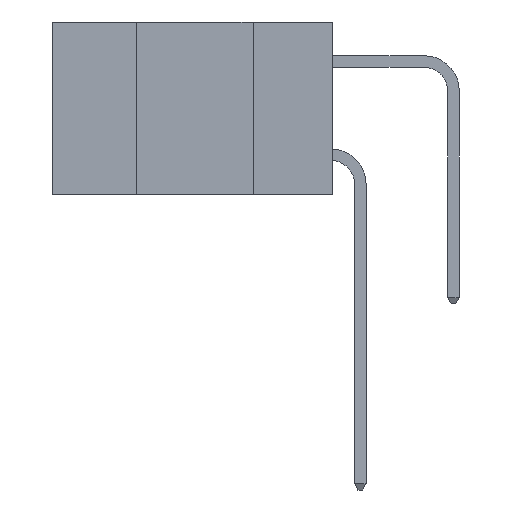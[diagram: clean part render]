
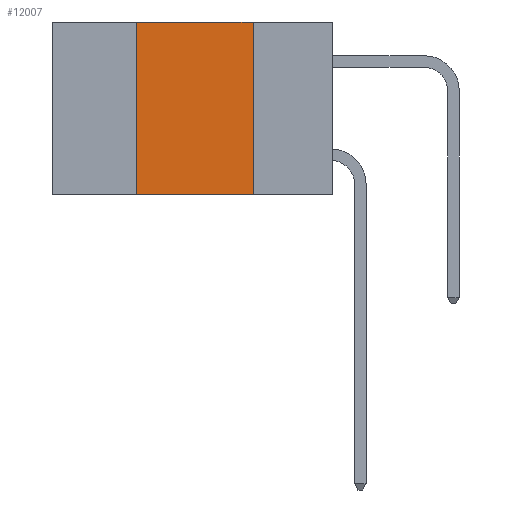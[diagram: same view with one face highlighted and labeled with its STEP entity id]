
A CAD part, left-side view. The second image highlights one B-rep face of the part: STEP entity #12007.
In plain terms, the highlighted planar face has unit normal (-1, 0, 0).
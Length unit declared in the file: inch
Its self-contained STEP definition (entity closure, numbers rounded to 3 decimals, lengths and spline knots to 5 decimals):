
#163 = CARTESIAN_POINT ( 'NONE',  ( 0., 0.6, -0.37 ) ) ;
#1012 = CARTESIAN_POINT ( 'NONE',  ( 0., 0.6, 0. ) ) ;
#1221 = EDGE_CURVE ( 'NONE', #1996, #1354, #9362, .T. ) ;
#1354 = VERTEX_POINT ( 'NONE', #14664 ) ;
#1779 = EDGE_CURVE ( 'NONE', #16366, #1354, #15950, .T. ) ;
#1996 = VERTEX_POINT ( 'NONE', #16228 ) ;
#3517 = ORIENTED_EDGE ( 'NONE', *, *, #1779, .F. ) ;
#3814 = ORIENTED_EDGE ( 'NONE', *, *, #7384, .F. ) ;
#3928 = ORIENTED_EDGE ( 'NONE', *, *, #11610, .F. ) ;
#4019 = ORIENTED_EDGE ( 'NONE', *, *, #1221, .T. ) ;
#4072 = FACE_OUTER_BOUND ( 'NONE', #10618, .T. ) ;
#4876 = DIRECTION ( 'NONE',  ( 0., 0., 1. ) ) ;
#5224 = VECTOR ( 'NONE', #19522, 39.37008 ) ;
#5882 = VECTOR ( 'NONE', #5979, 39.37008 ) ;
#5979 = DIRECTION ( 'NONE',  ( 0., -1., 0. ) ) ;
#6007 = CARTESIAN_POINT ( 'NONE',  ( 0., 0.6, 0. ) ) ;
#6533 = AXIS2_PLACEMENT_3D ( 'NONE', #1012, #7305, #17918 ) ;
#7305 = DIRECTION ( 'NONE',  ( 1., 0., 0. ) ) ;
#7384 = EDGE_CURVE ( 'NONE', #15137, #16366, #14022, .T. ) ;
#9362 = LINE ( 'NONE', #163, #5224 ) ;
#9865 = CARTESIAN_POINT ( 'NONE',  ( 0., 0.17, 0. ) ) ;
#10618 = EDGE_LOOP ( 'NONE', ( #3517, #3814, #3928, #4019 ) ) ;
#11610 = EDGE_CURVE ( 'NONE', #1996, #15137, #18849, .T. ) ;
#11945 = VECTOR ( 'NONE', #18987, 39.37008 ) ;
#12007 = ADVANCED_FACE ( 'NONE', ( #4072 ), #16402, .F. ) ;
#14022 = LINE ( 'NONE', #6007, #5882 ) ;
#14664 = CARTESIAN_POINT ( 'NONE',  ( 0., 0.17, -0.37 ) ) ;
#15137 = VERTEX_POINT ( 'NONE', #16248 ) ;
#15548 = CARTESIAN_POINT ( 'NONE',  ( 0., 0.42, -0.37 ) ) ;
#15950 = LINE ( 'NONE', #19046, #11945 ) ;
#16228 = CARTESIAN_POINT ( 'NONE',  ( 0., 0.42, -0.37 ) ) ;
#16248 = CARTESIAN_POINT ( 'NONE',  ( 0., 0.42, 0. ) ) ;
#16366 = VERTEX_POINT ( 'NONE', #9865 ) ;
#16402 = PLANE ( 'NONE',  #6533 ) ;
#17918 = DIRECTION ( 'NONE',  ( 0., 0., -1. ) ) ;
#18849 = LINE ( 'NONE', #15548, #19316 ) ;
#18987 = DIRECTION ( 'NONE',  ( 0., 0., -1. ) ) ;
#19046 = CARTESIAN_POINT ( 'NONE',  ( 0., 0.17, -0.37 ) ) ;
#19316 = VECTOR ( 'NONE', #4876, 39.37008 ) ;
#19522 = DIRECTION ( 'NONE',  ( 0., -1., 0. ) ) ;
